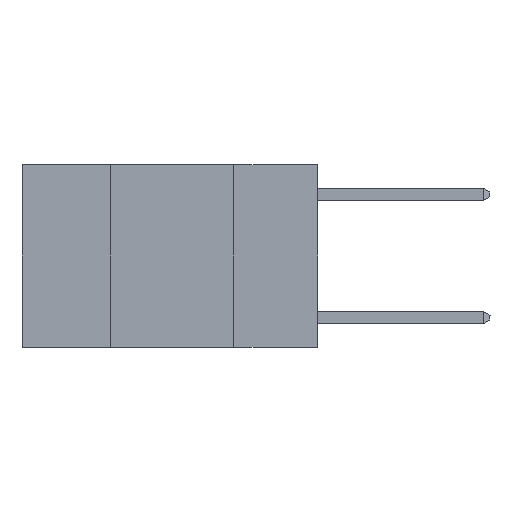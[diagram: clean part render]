
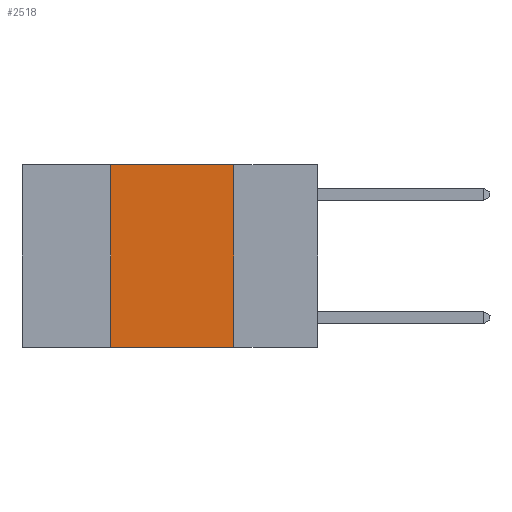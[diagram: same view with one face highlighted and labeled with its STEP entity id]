
A CAD part, left-side view. The second image highlights one B-rep face of the part: STEP entity #2518.
In plain terms, the highlighted planar face has unit normal (-1, 0, 0).
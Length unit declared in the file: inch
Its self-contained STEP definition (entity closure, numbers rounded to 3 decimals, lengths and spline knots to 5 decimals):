
#449 = DIRECTION ( 'NONE',  ( 1., 0., 0. ) ) ;
#1003 = CARTESIAN_POINT ( 'NONE',  ( 0., 0.6, -0.37 ) ) ;
#2064 = VERTEX_POINT ( 'NONE', #15638 ) ;
#2518 = ADVANCED_FACE ( 'NONE', ( #26393 ), #4535, .F. ) ;
#2544 = VERTEX_POINT ( 'NONE', #8698 ) ;
#4535 = PLANE ( 'NONE',  #5536 ) ;
#4915 = LINE ( 'NONE', #19962, #15336 ) ;
#5536 = AXIS2_PLACEMENT_3D ( 'NONE', #23169, #449, #14982 ) ;
#5982 = VECTOR ( 'NONE', #25749, 39.37008 ) ;
#6949 = CARTESIAN_POINT ( 'NONE',  ( 0., 0.42, 0. ) ) ;
#7335 = LINE ( 'NONE', #26185, #13528 ) ;
#7562 = CARTESIAN_POINT ( 'NONE',  ( 0., 0.42, -0.37 ) ) ;
#7793 = ORIENTED_EDGE ( 'NONE', *, *, #23439, .F. ) ;
#7964 = EDGE_CURVE ( 'NONE', #20715, #26227, #11501, .T. ) ;
#8698 = CARTESIAN_POINT ( 'NONE',  ( 0., 0.42, 0. ) ) ;
#11501 = LINE ( 'NONE', #1003, #5982 ) ;
#12030 = EDGE_CURVE ( 'NONE', #2064, #26227, #4915, .T. ) ;
#12677 = ORIENTED_EDGE ( 'NONE', *, *, #26660, .F. ) ;
#13528 = VECTOR ( 'NONE', #17961, 39.37008 ) ;
#13553 = VECTOR ( 'NONE', #19351, 39.37008 ) ;
#14221 = LINE ( 'NONE', #6949, #13553 ) ;
#14723 = EDGE_LOOP ( 'NONE', ( #23013, #12677, #7793, #18806 ) ) ;
#14982 = DIRECTION ( 'NONE',  ( 0., 0., -1. ) ) ;
#15336 = VECTOR ( 'NONE', #22043, 39.37008 ) ;
#15638 = CARTESIAN_POINT ( 'NONE',  ( 0., 0.17, 0. ) ) ;
#17961 = DIRECTION ( 'NONE',  ( 0., -1., 0. ) ) ;
#18806 = ORIENTED_EDGE ( 'NONE', *, *, #7964, .T. ) ;
#19351 = DIRECTION ( 'NONE',  ( 0., 0., 1. ) ) ;
#19962 = CARTESIAN_POINT ( 'NONE',  ( 0., 0.17, 0. ) ) ;
#20422 = CARTESIAN_POINT ( 'NONE',  ( 0., 0.17, -0.37 ) ) ;
#20715 = VERTEX_POINT ( 'NONE', #7562 ) ;
#22043 = DIRECTION ( 'NONE',  ( 0., 0., -1. ) ) ;
#23013 = ORIENTED_EDGE ( 'NONE', *, *, #12030, .F. ) ;
#23169 = CARTESIAN_POINT ( 'NONE',  ( 0., 0.6, 0. ) ) ;
#23439 = EDGE_CURVE ( 'NONE', #20715, #2544, #14221, .T. ) ;
#25749 = DIRECTION ( 'NONE',  ( 0., -1., 0. ) ) ;
#26185 = CARTESIAN_POINT ( 'NONE',  ( 0., 0.6, 0. ) ) ;
#26227 = VERTEX_POINT ( 'NONE', #20422 ) ;
#26393 = FACE_OUTER_BOUND ( 'NONE', #14723, .T. ) ;
#26660 = EDGE_CURVE ( 'NONE', #2544, #2064, #7335, .T. ) ;
